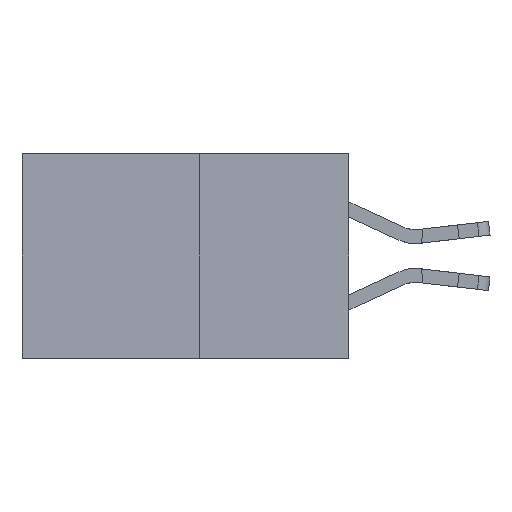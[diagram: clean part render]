
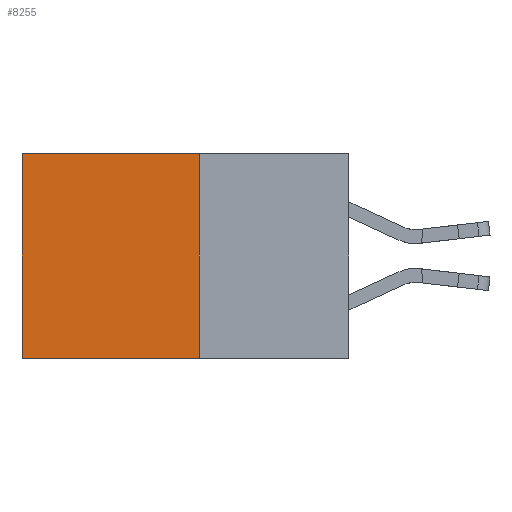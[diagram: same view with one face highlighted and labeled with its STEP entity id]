
A CAD part, left-side view. The second image highlights one B-rep face of the part: STEP entity #8255.
In plain terms, the highlighted planar face has unit normal (-1, 0, 0).
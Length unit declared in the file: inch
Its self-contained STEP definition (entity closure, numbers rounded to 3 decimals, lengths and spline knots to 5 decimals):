
#253 = ORIENTED_EDGE ( 'NONE', *, *, #4541, .F. ) ;
#434 = EDGE_LOOP ( 'NONE', ( #7465, #741, #253, #5755 ) ) ;
#741 = ORIENTED_EDGE ( 'NONE', *, *, #17191, .F. ) ;
#1408 = VECTOR ( 'NONE', #6036, 39.37008 ) ;
#1439 = VERTEX_POINT ( 'NONE', #15859 ) ;
#4332 = PLANE ( 'NONE',  #13729 ) ;
#4378 = VECTOR ( 'NONE', #4843, 39.37008 ) ;
#4541 = EDGE_CURVE ( 'NONE', #9255, #1439, #16990, .T. ) ;
#4581 = CARTESIAN_POINT ( 'NONE',  ( 0.277, 0.59, -0.37 ) ) ;
#4843 = DIRECTION ( 'NONE',  ( 0., 1., 0. ) ) ;
#5024 = CARTESIAN_POINT ( 'NONE',  ( 0.277, 0.27, 0. ) ) ;
#5410 = LINE ( 'NONE', #4581, #1408 ) ;
#5755 = ORIENTED_EDGE ( 'NONE', *, *, #12475, .T. ) ;
#5877 = DIRECTION ( 'NONE',  ( 0., 0., -1. ) ) ;
#6036 = DIRECTION ( 'NONE',  ( 0., 0., -1. ) ) ;
#6213 = CARTESIAN_POINT ( 'NONE',  ( 0.277, 0.27, -0.37 ) ) ;
#6454 = DIRECTION ( 'NONE',  ( 0., 1., 0. ) ) ;
#6490 = VECTOR ( 'NONE', #10404, 39.37008 ) ;
#7465 = ORIENTED_EDGE ( 'NONE', *, *, #14223, .T. ) ;
#8255 = ADVANCED_FACE ( 'NONE', ( #12522 ), #4332, .F. ) ;
#8360 = CARTESIAN_POINT ( 'NONE',  ( 0.277, 0.59, 0. ) ) ;
#9253 = VECTOR ( 'NONE', #6454, 39.37008 ) ;
#9255 = VERTEX_POINT ( 'NONE', #10304 ) ;
#9542 = CARTESIAN_POINT ( 'NONE',  ( 0.277, 0.59, -0.37 ) ) ;
#10153 = CARTESIAN_POINT ( 'NONE',  ( 0.277, 0.27, -0.37 ) ) ;
#10304 = CARTESIAN_POINT ( 'NONE',  ( 0.277, 0.27, 0. ) ) ;
#10404 = DIRECTION ( 'NONE',  ( 0., 0., -1. ) ) ;
#10692 = CARTESIAN_POINT ( 'NONE',  ( 0.277, 0.27, -0.37 ) ) ;
#11836 = VERTEX_POINT ( 'NONE', #9542 ) ;
#12475 = EDGE_CURVE ( 'NONE', #9255, #14003, #13550, .T. ) ;
#12489 = LINE ( 'NONE', #6213, #4378 ) ;
#12522 = FACE_OUTER_BOUND ( 'NONE', #434, .T. ) ;
#13550 = LINE ( 'NONE', #5024, #9253 ) ;
#13729 = AXIS2_PLACEMENT_3D ( 'NONE', #10153, #14452, #5877 ) ;
#14003 = VERTEX_POINT ( 'NONE', #8360 ) ;
#14223 = EDGE_CURVE ( 'NONE', #14003, #11836, #5410, .T. ) ;
#14452 = DIRECTION ( 'NONE',  ( 1., 0., 0. ) ) ;
#15859 = CARTESIAN_POINT ( 'NONE',  ( 0.277, 0.27, -0.37 ) ) ;
#16990 = LINE ( 'NONE', #10692, #6490 ) ;
#17191 = EDGE_CURVE ( 'NONE', #1439, #11836, #12489, .T. ) ;
